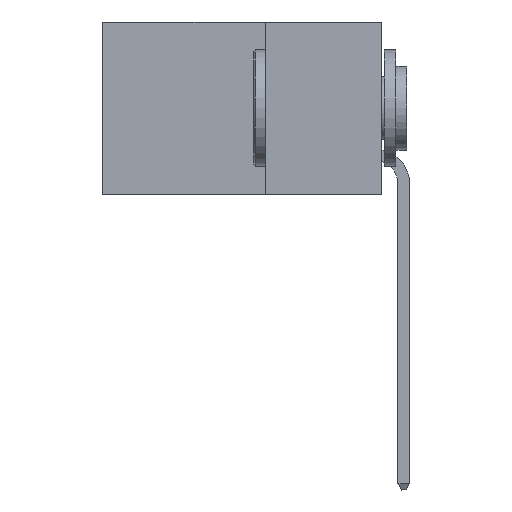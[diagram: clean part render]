
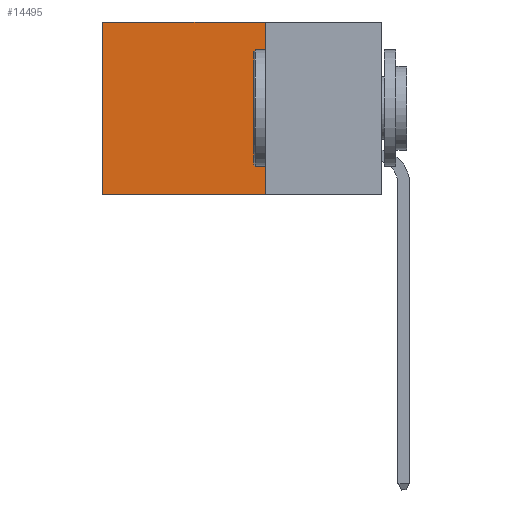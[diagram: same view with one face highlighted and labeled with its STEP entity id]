
A CAD part, left-side view. The second image highlights one B-rep face of the part: STEP entity #14495.
In plain terms, the highlighted planar face has unit normal (-1, 0, 0).
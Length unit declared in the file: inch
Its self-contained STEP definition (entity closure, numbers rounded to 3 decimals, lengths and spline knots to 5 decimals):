
#10 = DIRECTION ( 'NONE',  ( 0., 0., -1. ) ) ;
#1125 = ORIENTED_EDGE ( 'NONE', *, *, #4277, .F. ) ;
#4277 = EDGE_CURVE ( 'NONE', #26300, #31540, #6594, .T. ) ;
#4486 = DIRECTION ( 'NONE',  ( 0., 1., 0. ) ) ;
#5587 = DIRECTION ( 'NONE',  ( 1., 0., 0. ) ) ;
#5657 = VECTOR ( 'NONE', #16207, 39.37008 ) ;
#6482 = CARTESIAN_POINT ( 'NONE',  ( 0.2875, 0.25, -0.37 ) ) ;
#6594 = LINE ( 'NONE', #27849, #5657 ) ;
#6722 = EDGE_CURVE ( 'NONE', #26300, #15846, #21879, .T. ) ;
#8119 = EDGE_LOOP ( 'NONE', ( #15577, #15565, #1125, #15167 ) ) ;
#8457 = CARTESIAN_POINT ( 'NONE',  ( 0.2875, 0.25, 0. ) ) ;
#8934 = FACE_OUTER_BOUND ( 'NONE', #8119, .T. ) ;
#9731 = EDGE_CURVE ( 'NONE', #31540, #27024, #23944, .T. ) ;
#11233 = CARTESIAN_POINT ( 'NONE',  ( 0.2875, 0.25, -0.37 ) ) ;
#12353 = DIRECTION ( 'NONE',  ( 0., 1., 0. ) ) ;
#13264 = VECTOR ( 'NONE', #12353, 39.37008 ) ;
#14419 = DIRECTION ( 'NONE',  ( 0., 0., -1. ) ) ;
#14495 = ADVANCED_FACE ( 'NONE', ( #8934 ), #23394, .F. ) ;
#15167 = ORIENTED_EDGE ( 'NONE', *, *, #6722, .T. ) ;
#15565 = ORIENTED_EDGE ( 'NONE', *, *, #9731, .F. ) ;
#15577 = ORIENTED_EDGE ( 'NONE', *, *, #37257, .T. ) ;
#15846 = VERTEX_POINT ( 'NONE', #32114 ) ;
#16207 = DIRECTION ( 'NONE',  ( 0., 0., -1. ) ) ;
#17886 = CARTESIAN_POINT ( 'NONE',  ( 0.2875, 0.6, 0. ) ) ;
#19266 = CARTESIAN_POINT ( 'NONE',  ( 0.2875, 0.6, -0.37 ) ) ;
#21879 = LINE ( 'NONE', #38360, #32038 ) ;
#23394 = PLANE ( 'NONE',  #35080 ) ;
#23944 = LINE ( 'NONE', #6482, #13264 ) ;
#26300 = VERTEX_POINT ( 'NONE', #35983 ) ;
#27024 = VERTEX_POINT ( 'NONE', #19266 ) ;
#27849 = CARTESIAN_POINT ( 'NONE',  ( 0.2875, 0.25, 0. ) ) ;
#31540 = VERTEX_POINT ( 'NONE', #11233 ) ;
#32038 = VECTOR ( 'NONE', #4486, 39.37008 ) ;
#32114 = CARTESIAN_POINT ( 'NONE',  ( 0.2875, 0.6, 0. ) ) ;
#32477 = LINE ( 'NONE', #17886, #37556 ) ;
#35080 = AXIS2_PLACEMENT_3D ( 'NONE', #8457, #5587, #14419 ) ;
#35983 = CARTESIAN_POINT ( 'NONE',  ( 0.2875, 0.25, 0. ) ) ;
#37257 = EDGE_CURVE ( 'NONE', #15846, #27024, #32477, .T. ) ;
#37556 = VECTOR ( 'NONE', #10, 39.37008 ) ;
#38360 = CARTESIAN_POINT ( 'NONE',  ( 0.2875, 0.25, 0. ) ) ;
